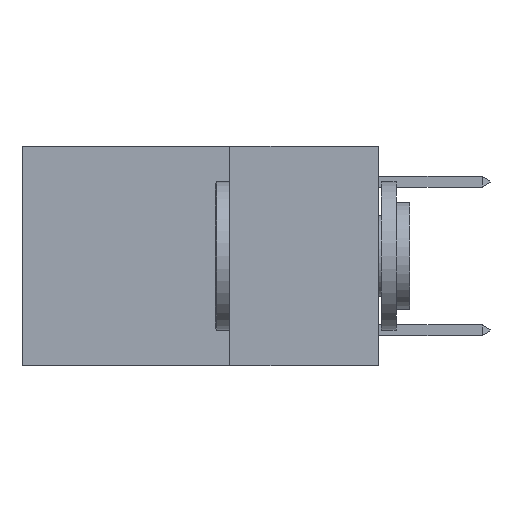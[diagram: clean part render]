
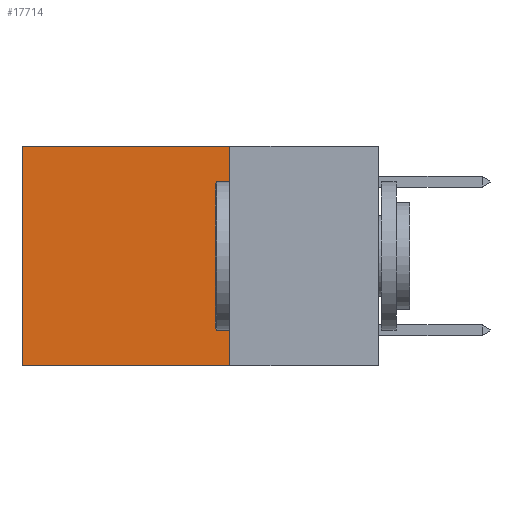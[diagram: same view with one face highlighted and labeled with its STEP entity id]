
A CAD part, left-side view. The second image highlights one B-rep face of the part: STEP entity #17714.
In plain terms, the highlighted planar face has unit normal (-1, 0, 0).
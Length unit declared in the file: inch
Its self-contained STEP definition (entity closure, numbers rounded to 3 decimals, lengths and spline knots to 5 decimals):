
#895 = VERTEX_POINT ( 'NONE', #16690 ) ;
#965 = CARTESIAN_POINT ( 'NONE',  ( 0.2625, 0.25, 0. ) ) ;
#3560 = AXIS2_PLACEMENT_3D ( 'NONE', #14444, #22311, #8022 ) ;
#3796 = DIRECTION ( 'NONE',  ( 0., 1., 0. ) ) ;
#4639 = EDGE_CURVE ( 'NONE', #20071, #8814, #6201, .T. ) ;
#4690 = DIRECTION ( 'NONE',  ( 0., 0., -1. ) ) ;
#5518 = CARTESIAN_POINT ( 'NONE',  ( 0.2625, 0.25, 0. ) ) ;
#5628 = VERTEX_POINT ( 'NONE', #11582 ) ;
#5657 = CARTESIAN_POINT ( 'NONE',  ( 0.2625, 0.25, -0.37 ) ) ;
#5939 = EDGE_CURVE ( 'NONE', #8814, #5628, #18303, .T. ) ;
#6201 = LINE ( 'NONE', #965, #19061 ) ;
#7362 = PLANE ( 'NONE',  #3560 ) ;
#7617 = CARTESIAN_POINT ( 'NONE',  ( 0.2625, 0.25, -0.37 ) ) ;
#8022 = DIRECTION ( 'NONE',  ( 0., 0., -1. ) ) ;
#8041 = DIRECTION ( 'NONE',  ( 0., 0., -1. ) ) ;
#8600 = ORIENTED_EDGE ( 'NONE', *, *, #19667, .T. ) ;
#8814 = VERTEX_POINT ( 'NONE', #5657 ) ;
#9595 = VECTOR ( 'NONE', #3796, 39.37008 ) ;
#10179 = EDGE_LOOP ( 'NONE', ( #8600, #13389, #12656, #20741 ) ) ;
#11582 = CARTESIAN_POINT ( 'NONE',  ( 0.2625, 0.6, -0.37 ) ) ;
#12656 = ORIENTED_EDGE ( 'NONE', *, *, #4639, .F. ) ;
#12940 = VECTOR ( 'NONE', #21653, 39.37008 ) ;
#13389 = ORIENTED_EDGE ( 'NONE', *, *, #5939, .F. ) ;
#14444 = CARTESIAN_POINT ( 'NONE',  ( 0.2625, 0.25, 0. ) ) ;
#15222 = FACE_OUTER_BOUND ( 'NONE', #10179, .T. ) ;
#16690 = CARTESIAN_POINT ( 'NONE',  ( 0.2625, 0.6, 0. ) ) ;
#17714 = ADVANCED_FACE ( 'NONE', ( #15222 ), #7362, .F. ) ;
#18059 = LINE ( 'NONE', #5518, #12940 ) ;
#18303 = LINE ( 'NONE', #7617, #9595 ) ;
#19061 = VECTOR ( 'NONE', #8041, 39.37008 ) ;
#19667 = EDGE_CURVE ( 'NONE', #895, #5628, #22088, .T. ) ;
#20071 = VERTEX_POINT ( 'NONE', #22103 ) ;
#20598 = CARTESIAN_POINT ( 'NONE',  ( 0.2625, 0.6, 0. ) ) ;
#20741 = ORIENTED_EDGE ( 'NONE', *, *, #22504, .T. ) ;
#21653 = DIRECTION ( 'NONE',  ( 0., 1., 0. ) ) ;
#21845 = VECTOR ( 'NONE', #4690, 39.37008 ) ;
#22088 = LINE ( 'NONE', #20598, #21845 ) ;
#22103 = CARTESIAN_POINT ( 'NONE',  ( 0.2625, 0.25, 0. ) ) ;
#22311 = DIRECTION ( 'NONE',  ( 1., 0., 0. ) ) ;
#22504 = EDGE_CURVE ( 'NONE', #20071, #895, #18059, .T. ) ;
